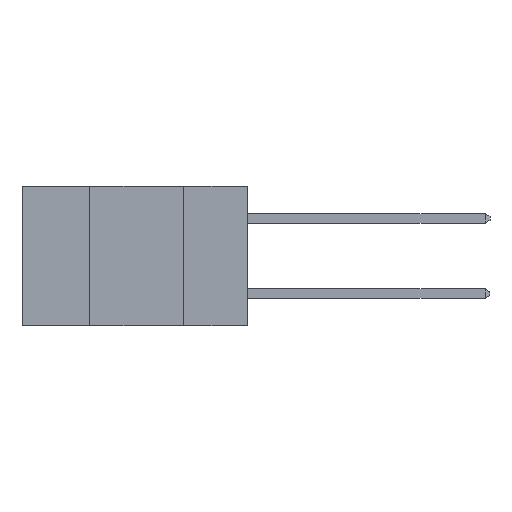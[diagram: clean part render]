
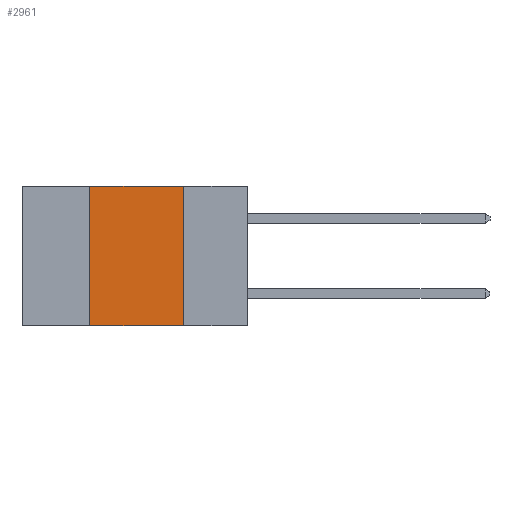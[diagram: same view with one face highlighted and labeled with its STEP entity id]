
A CAD part, left-side view. The second image highlights one B-rep face of the part: STEP entity #2961.
In plain terms, the highlighted planar face has unit normal (-1, 0, 0).
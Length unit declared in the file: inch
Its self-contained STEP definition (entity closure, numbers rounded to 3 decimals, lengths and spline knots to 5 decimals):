
#26 = VERTEX_POINT ( 'NONE', #2205 ) ;
#676 = VERTEX_POINT ( 'NONE', #3880 ) ;
#765 = VECTOR ( 'NONE', #2281, 39.37008 ) ;
#1102 = ORIENTED_EDGE ( 'NONE', *, *, #3191, .F. ) ;
#1291 = DIRECTION ( 'NONE',  ( 0., -1., 0. ) ) ;
#1645 = LINE ( 'NONE', #3288, #5175 ) ;
#2019 = EDGE_CURVE ( 'NONE', #8619, #26, #6527, .T. ) ;
#2205 = CARTESIAN_POINT ( 'NONE',  ( 0., 0.42, 0. ) ) ;
#2281 = DIRECTION ( 'NONE',  ( 0., 0., 1. ) ) ;
#2913 = CARTESIAN_POINT ( 'NONE',  ( 0., 0.6, 0. ) ) ;
#2932 = PLANE ( 'NONE',  #5985 ) ;
#2961 = ADVANCED_FACE ( 'NONE', ( #6613 ), #2932, .F. ) ;
#2982 = VECTOR ( 'NONE', #4642, 39.37008 ) ;
#3044 = DIRECTION ( 'NONE',  ( 0., -1., 0. ) ) ;
#3078 = EDGE_LOOP ( 'NONE', ( #4088, #1102, #7611, #5694 ) ) ;
#3191 = EDGE_CURVE ( 'NONE', #26, #4817, #8220, .T. ) ;
#3277 = EDGE_CURVE ( 'NONE', #8619, #676, #1645, .T. ) ;
#3288 = CARTESIAN_POINT ( 'NONE',  ( 0., 0.6, -0.37 ) ) ;
#3880 = CARTESIAN_POINT ( 'NONE',  ( 0., 0.17, -0.37 ) ) ;
#4088 = ORIENTED_EDGE ( 'NONE', *, *, #4658, .F. ) ;
#4642 = DIRECTION ( 'NONE',  ( 0., 0., -1. ) ) ;
#4658 = EDGE_CURVE ( 'NONE', #4817, #676, #6489, .T. ) ;
#4817 = VERTEX_POINT ( 'NONE', #7687 ) ;
#5175 = VECTOR ( 'NONE', #1291, 39.37008 ) ;
#5662 = CARTESIAN_POINT ( 'NONE',  ( 0., 0.42, 0. ) ) ;
#5694 = ORIENTED_EDGE ( 'NONE', *, *, #3277, .T. ) ;
#5792 = DIRECTION ( 'NONE',  ( 0., 0., -1. ) ) ;
#5806 = DIRECTION ( 'NONE',  ( 1., 0., 0. ) ) ;
#5985 = AXIS2_PLACEMENT_3D ( 'NONE', #2913, #5806, #5792 ) ;
#6221 = CARTESIAN_POINT ( 'NONE',  ( 0., 0.6, 0. ) ) ;
#6489 = LINE ( 'NONE', #6929, #2982 ) ;
#6527 = LINE ( 'NONE', #5662, #765 ) ;
#6613 = FACE_OUTER_BOUND ( 'NONE', #3078, .T. ) ;
#6929 = CARTESIAN_POINT ( 'NONE',  ( 0., 0.17, 0. ) ) ;
#7611 = ORIENTED_EDGE ( 'NONE', *, *, #2019, .F. ) ;
#7687 = CARTESIAN_POINT ( 'NONE',  ( 0., 0.17, 0. ) ) ;
#7986 = VECTOR ( 'NONE', #3044, 39.37008 ) ;
#8220 = LINE ( 'NONE', #6221, #7986 ) ;
#8308 = CARTESIAN_POINT ( 'NONE',  ( 0., 0.42, -0.37 ) ) ;
#8619 = VERTEX_POINT ( 'NONE', #8308 ) ;
